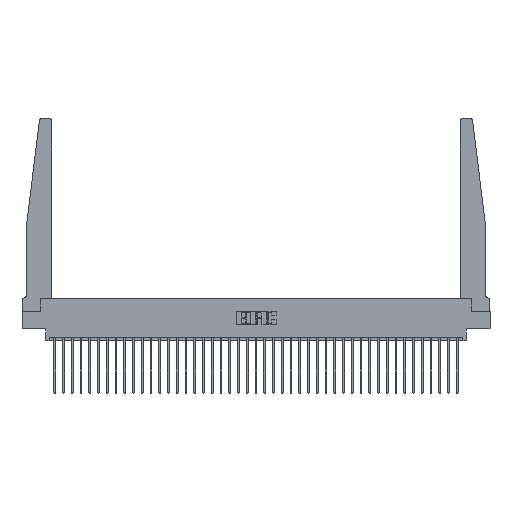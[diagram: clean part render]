
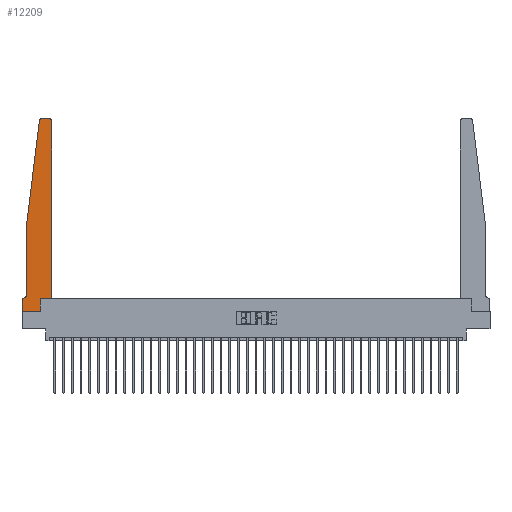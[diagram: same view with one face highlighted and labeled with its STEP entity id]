
A CAD part, top view. The second image highlights one B-rep face of the part: STEP entity #12209.
In plain terms, the highlighted planar face has unit normal (0, 0, 1).
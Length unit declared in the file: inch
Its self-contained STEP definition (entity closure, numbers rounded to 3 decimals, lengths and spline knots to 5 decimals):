
#366 = CARTESIAN_POINT ( 'NONE',  ( 0.2605, 0.18, 0.37 ) ) ;
#394 = LINE ( 'NONE', #27271, #12283 ) ;
#870 = DIRECTION ( 'NONE',  ( -1., 0., 0. ) ) ;
#1206 = CARTESIAN_POINT ( 'NONE',  ( 0.25, 2.75, 0.37 ) ) ;
#2587 = CIRCLE ( 'NONE', #18578, 0.03 ) ;
#2788 = DIRECTION ( 'NONE',  ( 0., 1., 0. ) ) ;
#3029 = CARTESIAN_POINT ( 'NONE',  ( 0., 0., 0.37 ) ) ;
#3510 = CARTESIAN_POINT ( 'NONE',  ( 0.24675, 2.72367, 0.37 ) ) ;
#3847 = AXIS2_PLACEMENT_3D ( 'NONE', #29744, #5208, #16117 ) ;
#4062 = DIRECTION ( 'NONE',  ( -1., 0., 0. ) ) ;
#4079 = VERTEX_POINT ( 'NONE', #21312 ) ;
#4643 = EDGE_CURVE ( 'NONE', #15203, #26295, #24985, .T. ) ;
#5208 = DIRECTION ( 'NONE',  ( 0., 0., 1. ) ) ;
#5528 = CARTESIAN_POINT ( 'NONE',  ( 0.015, 0.1875, 0.37 ) ) ;
#6029 = LINE ( 'NONE', #1206, #22231 ) ;
#6587 = DIRECTION ( 'NONE',  ( 0., 0., 1. ) ) ;
#7310 = EDGE_CURVE ( 'NONE', #19613, #4079, #13880, .T. ) ;
#8223 = CARTESIAN_POINT ( 'NONE',  ( 0.27653, 2.75, 0.37 ) ) ;
#8320 = DIRECTION ( 'NONE',  ( 0., -1., 0. ) ) ;
#8324 = ORIENTED_EDGE ( 'NONE', *, *, #29729, .T. ) ;
#8487 = CARTESIAN_POINT ( 'NONE',  ( 0.065, 1.25, 0.37 ) ) ;
#8534 = CARTESIAN_POINT ( 'NONE',  ( 0.425, 2.72, 0.37 ) ) ;
#9258 = VERTEX_POINT ( 'NONE', #9294 ) ;
#9267 = EDGE_LOOP ( 'NONE', ( #34391, #18693, #30793, #27066, #19939, #20336, #12750, #11045, #25895, #8324, #29718, #31397 ) ) ;
#9294 = CARTESIAN_POINT ( 'NONE',  ( 0.425, 0.18, 0.37 ) ) ;
#9444 = CARTESIAN_POINT ( 'NONE',  ( 0.015, 0.2375, 0.37 ) ) ;
#9534 = VERTEX_POINT ( 'NONE', #5528 ) ;
#9721 = CARTESIAN_POINT ( 'NONE',  ( 0., 0.1875, 0.37 ) ) ;
#10003 = AXIS2_PLACEMENT_3D ( 'NONE', #9444, #17148, #870 ) ;
#10861 = VERTEX_POINT ( 'NONE', #8223 ) ;
#11045 = ORIENTED_EDGE ( 'NONE', *, *, #7310, .T. ) ;
#11139 = CARTESIAN_POINT ( 'NONE',  ( 0., 0., 0.37 ) ) ;
#11310 = VERTEX_POINT ( 'NONE', #9721 ) ;
#12209 = ADVANCED_FACE ( 'NONE', ( #22898 ), #34010, .T. ) ;
#12283 = VECTOR ( 'NONE', #24413, 39.37008 ) ;
#12520 = VERTEX_POINT ( 'NONE', #3510 ) ;
#12750 = ORIENTED_EDGE ( 'NONE', *, *, #28562, .T. ) ;
#12864 = EDGE_CURVE ( 'NONE', #9258, #20532, #16024, .T. ) ;
#13210 = CARTESIAN_POINT ( 'NONE',  ( 0.065, 0.2375, 0.37 ) ) ;
#13463 = VECTOR ( 'NONE', #24900, 39.37008 ) ;
#13880 = LINE ( 'NONE', #22991, #23125 ) ;
#15203 = VERTEX_POINT ( 'NONE', #28705 ) ;
#16024 = LINE ( 'NONE', #16204, #18397 ) ;
#16117 = DIRECTION ( 'NONE',  ( 1., 0., 0. ) ) ;
#16204 = CARTESIAN_POINT ( 'NONE',  ( 0.425, 0.18, 0.37 ) ) ;
#16575 = EDGE_CURVE ( 'NONE', #20532, #32390, #2587, .T. ) ;
#16685 = EDGE_CURVE ( 'NONE', #4079, #33261, #394, .T. ) ;
#17148 = DIRECTION ( 'NONE',  ( 0., 0., -1. ) ) ;
#17232 = EDGE_CURVE ( 'NONE', #9534, #11310, #22186, .T. ) ;
#18033 = EDGE_CURVE ( 'NONE', #12520, #15203, #27280, .T. ) ;
#18397 = VECTOR ( 'NONE', #2788, 39.37008 ) ;
#18578 = AXIS2_PLACEMENT_3D ( 'NONE', #31756, #26736, #28898 ) ;
#18693 = ORIENTED_EDGE ( 'NONE', *, *, #33352, .T. ) ;
#18833 = LINE ( 'NONE', #32270, #25409 ) ;
#19046 = AXIS2_PLACEMENT_3D ( 'NONE', #20206, #6587, #28455 ) ;
#19293 = CIRCLE ( 'NONE', #3847, 0.03 ) ;
#19613 = VERTEX_POINT ( 'NONE', #11139 ) ;
#19939 = ORIENTED_EDGE ( 'NONE', *, *, #28722, .T. ) ;
#20206 = CARTESIAN_POINT ( 'NONE',  ( 0., 0.1875, 0.37 ) ) ;
#20336 = ORIENTED_EDGE ( 'NONE', *, *, #17232, .T. ) ;
#20532 = VERTEX_POINT ( 'NONE', #8534 ) ;
#21312 = CARTESIAN_POINT ( 'NONE',  ( 0.2605, 0., 0.37 ) ) ;
#21935 = CARTESIAN_POINT ( 'NONE',  ( 0.395, 2.75, 0.37 ) ) ;
#22175 = LINE ( 'NONE', #3029, #26607 ) ;
#22186 = LINE ( 'NONE', #27572, #13463 ) ;
#22231 = VECTOR ( 'NONE', #4062, 39.37008 ) ;
#22291 = DIRECTION ( 'NONE',  ( 1., 0., 0. ) ) ;
#22898 = FACE_OUTER_BOUND ( 'NONE', #9267, .T. ) ;
#22991 = CARTESIAN_POINT ( 'NONE',  ( 0., 0., 0.37 ) ) ;
#23125 = VECTOR ( 'NONE', #22291, 39.37008 ) ;
#24237 = CARTESIAN_POINT ( 'NONE',  ( 0.065, 1.25, 0.37 ) ) ;
#24413 = DIRECTION ( 'NONE',  ( 0., 1., 0. ) ) ;
#24774 = DIRECTION ( 'NONE',  ( -0.122, -0.992, 0. ) ) ;
#24900 = DIRECTION ( 'NONE',  ( -1., 0., 0. ) ) ;
#24985 = LINE ( 'NONE', #8487, #27581 ) ;
#25156 = EDGE_CURVE ( 'NONE', #32390, #10861, #6029, .T. ) ;
#25409 = VECTOR ( 'NONE', #27269, 39.37008 ) ;
#25437 = CIRCLE ( 'NONE', #10003, 0.05 ) ;
#25895 = ORIENTED_EDGE ( 'NONE', *, *, #16685, .T. ) ;
#26295 = VERTEX_POINT ( 'NONE', #13210 ) ;
#26607 = VECTOR ( 'NONE', #29723, 39.37008 ) ;
#26736 = DIRECTION ( 'NONE',  ( 0., 0., 1. ) ) ;
#27006 = VECTOR ( 'NONE', #24774, 39.37008 ) ;
#27066 = ORIENTED_EDGE ( 'NONE', *, *, #4643, .T. ) ;
#27269 = DIRECTION ( 'NONE',  ( 1., 0., 0. ) ) ;
#27271 = CARTESIAN_POINT ( 'NONE',  ( 0.2605, 0.18, 0.37 ) ) ;
#27280 = LINE ( 'NONE', #24237, #27006 ) ;
#27572 = CARTESIAN_POINT ( 'NONE',  ( 0.065, 0.1875, 0.37 ) ) ;
#27581 = VECTOR ( 'NONE', #8320, 39.37008 ) ;
#28455 = DIRECTION ( 'NONE',  ( 1., 0., 0. ) ) ;
#28562 = EDGE_CURVE ( 'NONE', #11310, #19613, #22175, .T. ) ;
#28705 = CARTESIAN_POINT ( 'NONE',  ( 0.065, 1.25, 0.37 ) ) ;
#28722 = EDGE_CURVE ( 'NONE', #26295, #9534, #25437, .T. ) ;
#28898 = DIRECTION ( 'NONE',  ( 1., 0., 0. ) ) ;
#29718 = ORIENTED_EDGE ( 'NONE', *, *, #12864, .T. ) ;
#29723 = DIRECTION ( 'NONE',  ( 0., -1., 0. ) ) ;
#29729 = EDGE_CURVE ( 'NONE', #33261, #9258, #18833, .T. ) ;
#29744 = CARTESIAN_POINT ( 'NONE',  ( 0.27653, 2.72, 0.37 ) ) ;
#30793 = ORIENTED_EDGE ( 'NONE', *, *, #18033, .T. ) ;
#31397 = ORIENTED_EDGE ( 'NONE', *, *, #16575, .T. ) ;
#31756 = CARTESIAN_POINT ( 'NONE',  ( 0.395, 2.72, 0.37 ) ) ;
#32270 = CARTESIAN_POINT ( 'NONE',  ( 0.425, 0.18, 0.37 ) ) ;
#32390 = VERTEX_POINT ( 'NONE', #21935 ) ;
#33261 = VERTEX_POINT ( 'NONE', #366 ) ;
#33352 = EDGE_CURVE ( 'NONE', #10861, #12520, #19293, .T. ) ;
#34010 = PLANE ( 'NONE',  #19046 ) ;
#34391 = ORIENTED_EDGE ( 'NONE', *, *, #25156, .T. ) ;
